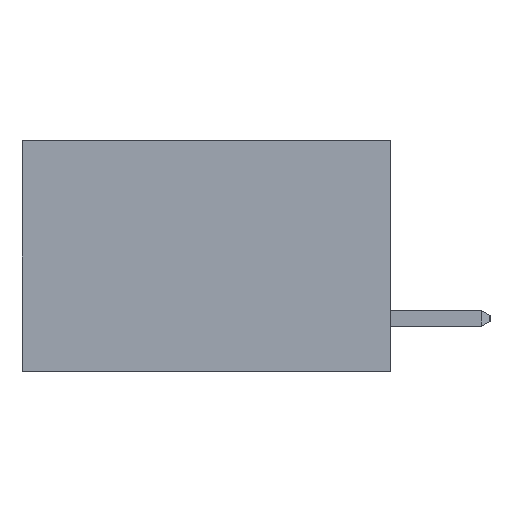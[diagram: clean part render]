
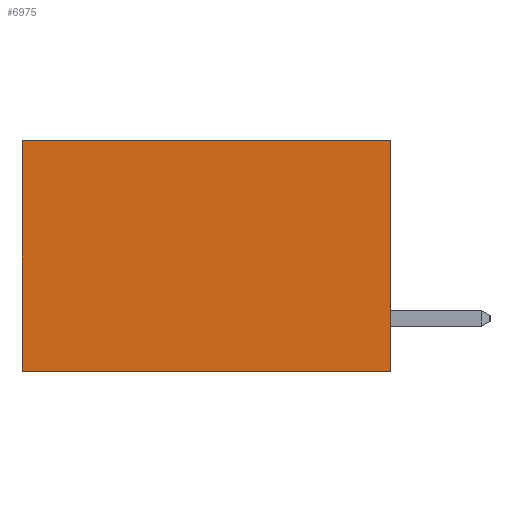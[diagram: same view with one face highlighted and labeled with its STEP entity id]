
A CAD part, left-side view. The second image highlights one B-rep face of the part: STEP entity #6975.
In plain terms, the highlighted planar face has unit normal (-1, 0, 0).
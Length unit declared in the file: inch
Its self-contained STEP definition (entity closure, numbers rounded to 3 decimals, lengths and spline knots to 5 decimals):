
#145 = DIRECTION ( 'NONE',  ( 0., 0., -1. ) ) ;
#219 = CARTESIAN_POINT ( 'NONE',  ( 0.277, 0.59, -0.37 ) ) ;
#524 = EDGE_CURVE ( 'NONE', #8339, #4438, #9028, .T. ) ;
#929 = EDGE_CURVE ( 'NONE', #5510, #11905, #8618, .T. ) ;
#1779 = ORIENTED_EDGE ( 'NONE', *, *, #9182, .T. ) ;
#2200 = LINE ( 'NONE', #6852, #6015 ) ;
#2513 = FACE_OUTER_BOUND ( 'NONE', #13334, .T. ) ;
#3407 = AXIS2_PLACEMENT_3D ( 'NONE', #4671, #4599, #4595 ) ;
#3599 = DIRECTION ( 'NONE',  ( 0., 1., 0. ) ) ;
#4438 = VERTEX_POINT ( 'NONE', #6635 ) ;
#4490 = EDGE_CURVE ( 'NONE', #5510, #8339, #2200, .T. ) ;
#4595 = DIRECTION ( 'NONE',  ( 0., 0., -1. ) ) ;
#4599 = DIRECTION ( 'NONE',  ( 1., 0., 0. ) ) ;
#4616 = PLANE ( 'NONE',  #3407 ) ;
#4671 = CARTESIAN_POINT ( 'NONE',  ( 0.277, 0., -0.37 ) ) ;
#4802 = DIRECTION ( 'NONE',  ( 0., 0., -1. ) ) ;
#5009 = DIRECTION ( 'NONE',  ( 0., 1., 0. ) ) ;
#5081 = CARTESIAN_POINT ( 'NONE',  ( 0.277, 0., -0.37 ) ) ;
#5510 = VERTEX_POINT ( 'NONE', #11141 ) ;
#5636 = CARTESIAN_POINT ( 'NONE',  ( 0.277, 0., 0. ) ) ;
#6015 = VECTOR ( 'NONE', #4802, 39.37008 ) ;
#6635 = CARTESIAN_POINT ( 'NONE',  ( 0.277, 0.59, -0.37 ) ) ;
#6852 = CARTESIAN_POINT ( 'NONE',  ( 0.277, 0., -0.37 ) ) ;
#6975 = ADVANCED_FACE ( 'NONE', ( #2513 ), #4616, .F. ) ;
#8339 = VERTEX_POINT ( 'NONE', #12507 ) ;
#8536 = LINE ( 'NONE', #219, #11412 ) ;
#8618 = LINE ( 'NONE', #5636, #14690 ) ;
#8810 = CARTESIAN_POINT ( 'NONE',  ( 0.277, 0.59, 0. ) ) ;
#9028 = LINE ( 'NONE', #5081, #12244 ) ;
#9182 = EDGE_CURVE ( 'NONE', #11905, #4438, #8536, .T. ) ;
#10974 = ORIENTED_EDGE ( 'NONE', *, *, #524, .F. ) ;
#11141 = CARTESIAN_POINT ( 'NONE',  ( 0.277, 0., 0. ) ) ;
#11412 = VECTOR ( 'NONE', #145, 39.37008 ) ;
#11905 = VERTEX_POINT ( 'NONE', #8810 ) ;
#12048 = ORIENTED_EDGE ( 'NONE', *, *, #929, .T. ) ;
#12244 = VECTOR ( 'NONE', #5009, 39.37008 ) ;
#12507 = CARTESIAN_POINT ( 'NONE',  ( 0.277, 0., -0.37 ) ) ;
#13334 = EDGE_LOOP ( 'NONE', ( #1779, #10974, #15609, #12048 ) ) ;
#14690 = VECTOR ( 'NONE', #3599, 39.37008 ) ;
#15609 = ORIENTED_EDGE ( 'NONE', *, *, #4490, .F. ) ;
